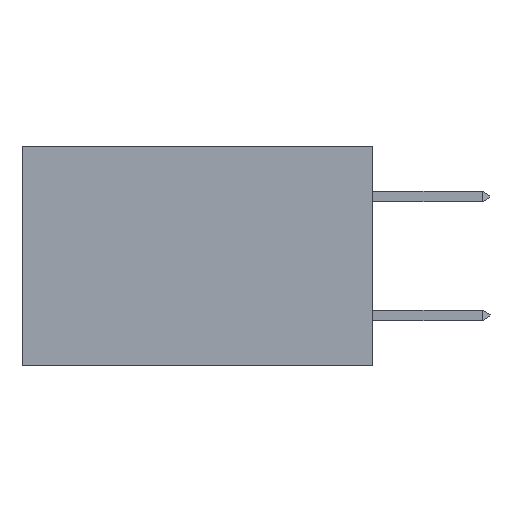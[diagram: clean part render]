
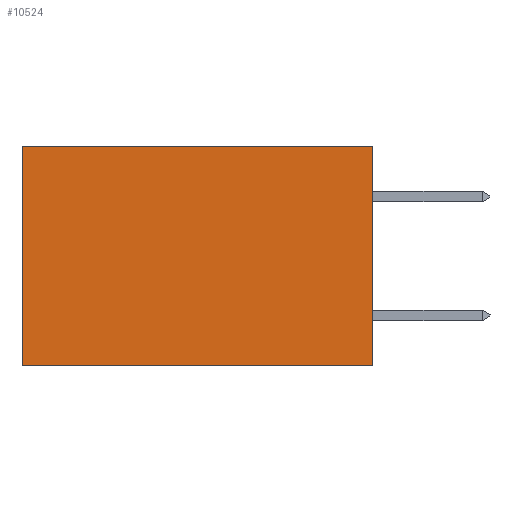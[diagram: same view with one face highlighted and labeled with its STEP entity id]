
A CAD part, left-side view. The second image highlights one B-rep face of the part: STEP entity #10524.
In plain terms, the highlighted planar face has unit normal (-1, 0, 0).
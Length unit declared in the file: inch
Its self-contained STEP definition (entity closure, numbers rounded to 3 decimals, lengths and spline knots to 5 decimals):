
#98 = EDGE_CURVE ( 'NONE', #14556, #18888, #19274, .T. ) ;
#1447 = EDGE_LOOP ( 'NONE', ( #25592, #17333, #22165, #12534 ) ) ;
#1969 = CARTESIAN_POINT ( 'NONE',  ( 0.277, 0.59, -0.37 ) ) ;
#3189 = CARTESIAN_POINT ( 'NONE',  ( 0.277, 0., 0. ) ) ;
#3804 = VECTOR ( 'NONE', #19940, 39.37008 ) ;
#5663 = CARTESIAN_POINT ( 'NONE',  ( 0.277, 0., 0. ) ) ;
#5989 = LINE ( 'NONE', #23309, #10943 ) ;
#6124 = DIRECTION ( 'NONE',  ( 0., 0., -1. ) ) ;
#6142 = VERTEX_POINT ( 'NONE', #1969 ) ;
#7231 = EDGE_CURVE ( 'NONE', #14556, #18129, #5989, .T. ) ;
#7237 = FACE_OUTER_BOUND ( 'NONE', #1447, .T. ) ;
#10524 = ADVANCED_FACE ( 'NONE', ( #7237 ), #22896, .F. ) ;
#10943 = VECTOR ( 'NONE', #14216, 39.37008 ) ;
#11274 = DIRECTION ( 'NONE',  ( 0., 1., 0. ) ) ;
#12534 = ORIENTED_EDGE ( 'NONE', *, *, #98, .T. ) ;
#12853 = AXIS2_PLACEMENT_3D ( 'NONE', #27161, #18750, #6124 ) ;
#14216 = DIRECTION ( 'NONE',  ( 0., 0., -1. ) ) ;
#14456 = DIRECTION ( 'NONE',  ( 0., 0., -1. ) ) ;
#14556 = VERTEX_POINT ( 'NONE', #3189 ) ;
#16264 = VECTOR ( 'NONE', #14456, 39.37008 ) ;
#16341 = EDGE_CURVE ( 'NONE', #18129, #6142, #22270, .T. ) ;
#16460 = CARTESIAN_POINT ( 'NONE',  ( 0.277, 0.59, -0.37 ) ) ;
#17333 = ORIENTED_EDGE ( 'NONE', *, *, #16341, .F. ) ;
#17865 = EDGE_CURVE ( 'NONE', #18888, #6142, #22512, .T. ) ;
#18129 = VERTEX_POINT ( 'NONE', #24116 ) ;
#18750 = DIRECTION ( 'NONE',  ( 1., 0., 0. ) ) ;
#18888 = VERTEX_POINT ( 'NONE', #20126 ) ;
#19274 = LINE ( 'NONE', #5663, #3804 ) ;
#19940 = DIRECTION ( 'NONE',  ( 0., 1., 0. ) ) ;
#20126 = CARTESIAN_POINT ( 'NONE',  ( 0.277, 0.59, 0. ) ) ;
#21610 = VECTOR ( 'NONE', #11274, 39.37008 ) ;
#21862 = CARTESIAN_POINT ( 'NONE',  ( 0.277, 0., -0.37 ) ) ;
#22165 = ORIENTED_EDGE ( 'NONE', *, *, #7231, .F. ) ;
#22270 = LINE ( 'NONE', #21862, #21610 ) ;
#22512 = LINE ( 'NONE', #16460, #16264 ) ;
#22896 = PLANE ( 'NONE',  #12853 ) ;
#23309 = CARTESIAN_POINT ( 'NONE',  ( 0.277, 0., -0.37 ) ) ;
#24116 = CARTESIAN_POINT ( 'NONE',  ( 0.277, 0., -0.37 ) ) ;
#25592 = ORIENTED_EDGE ( 'NONE', *, *, #17865, .T. ) ;
#27161 = CARTESIAN_POINT ( 'NONE',  ( 0.277, 0., -0.37 ) ) ;
